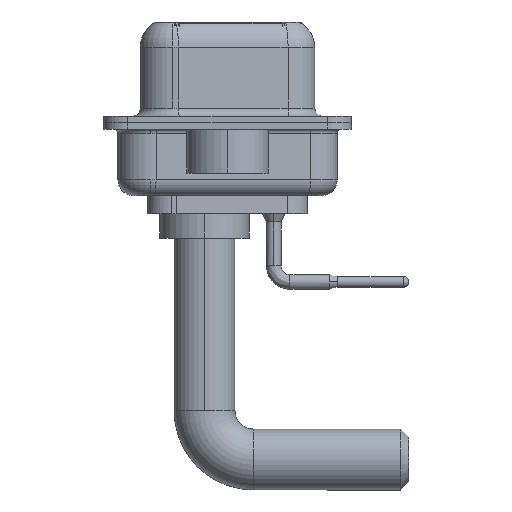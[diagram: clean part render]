
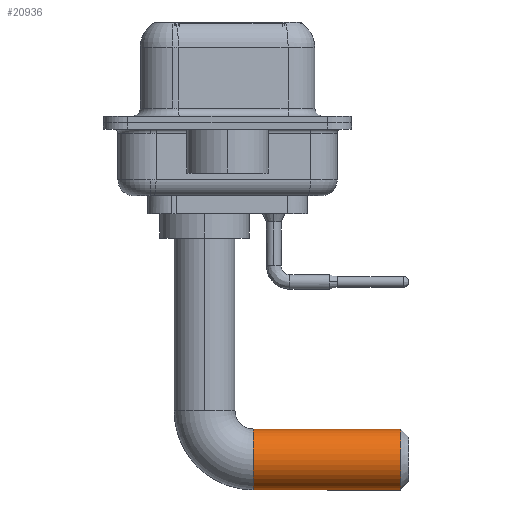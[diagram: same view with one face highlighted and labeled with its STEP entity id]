
A CAD part, left-side view. The second image highlights one B-rep face of the part: STEP entity #20936.
In plain terms, the highlighted cylindrical face has radius 1.875 mm (diameter 3.75 mm), a partial arc.
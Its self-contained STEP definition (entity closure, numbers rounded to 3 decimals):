
#50 = DIRECTION ( 'NONE',  ( -1., 0., 0. ) ) ;
#132 = EDGE_LOOP ( 'NONE', ( #13651, #15798, #13271, #6281 ) ) ;
#420 = CARTESIAN_POINT ( 'NONE',  ( 0., -3., -11.755 ) ) ;
#433 = LINE ( 'NONE', #12418, #16903 ) ;
#862 = AXIS2_PLACEMENT_3D ( 'NONE', #19703, #20893, #1698 ) ;
#1386 = CYLINDRICAL_SURFACE ( 'NONE', #862, 1.875 ) ;
#1459 = DIRECTION ( 'NONE',  ( 0., -1., 0. ) ) ;
#1698 = DIRECTION ( 'NONE',  ( 0., 0., -1. ) ) ;
#2107 = EDGE_CURVE ( 'NONE', #21097, #6196, #433, .T. ) ;
#2365 = EDGE_CURVE ( 'NONE', #9336, #9320, #11320, .T. ) ;
#3881 = CARTESIAN_POINT ( 'NONE',  ( 0., -12.07, -11.755 ) ) ;
#5141 = DIRECTION ( 'NONE',  ( 0., -1., 0. ) ) ;
#5563 = EDGE_CURVE ( 'NONE', #9320, #6196, #15329, .T. ) ;
#5795 = FACE_OUTER_BOUND ( 'NONE', #132, .T. ) ;
#6196 = VERTEX_POINT ( 'NONE', #3881 ) ;
#6281 = ORIENTED_EDGE ( 'NONE', *, *, #5563, .T. ) ;
#6403 = CIRCLE ( 'NONE', #9518, 1.875 ) ;
#9288 = CARTESIAN_POINT ( 'NONE',  ( 0., -3., -15.505 ) ) ;
#9320 = VERTEX_POINT ( 'NONE', #19049 ) ;
#9336 = VERTEX_POINT ( 'NONE', #9288 ) ;
#9518 = AXIS2_PLACEMENT_3D ( 'NONE', #14736, #9585, #50 ) ;
#9585 = DIRECTION ( 'NONE',  ( 0., -1., 0. ) ) ;
#10874 = AXIS2_PLACEMENT_3D ( 'NONE', #15949, #14142, #19469 ) ;
#11320 = LINE ( 'NONE', #16037, #14190 ) ;
#12178 = EDGE_CURVE ( 'NONE', #21097, #9336, #6403, .T. ) ;
#12418 = CARTESIAN_POINT ( 'NONE',  ( 0., -3., -11.755 ) ) ;
#13271 = ORIENTED_EDGE ( 'NONE', *, *, #2365, .T. ) ;
#13651 = ORIENTED_EDGE ( 'NONE', *, *, #2107, .F. ) ;
#14142 = DIRECTION ( 'NONE',  ( 0., 1., 0. ) ) ;
#14190 = VECTOR ( 'NONE', #1459, 1000. ) ;
#14736 = CARTESIAN_POINT ( 'NONE',  ( 0., -3., -13.63 ) ) ;
#15329 = CIRCLE ( 'NONE', #10874, 1.875 ) ;
#15798 = ORIENTED_EDGE ( 'NONE', *, *, #12178, .T. ) ;
#15949 = CARTESIAN_POINT ( 'NONE',  ( 0., -12.07, -13.63 ) ) ;
#16037 = CARTESIAN_POINT ( 'NONE',  ( 0., -3., -15.505 ) ) ;
#16903 = VECTOR ( 'NONE', #5141, 1000. ) ;
#19049 = CARTESIAN_POINT ( 'NONE',  ( 0., -12.07, -15.505 ) ) ;
#19469 = DIRECTION ( 'NONE',  ( 0., 0., -1. ) ) ;
#19703 = CARTESIAN_POINT ( 'NONE',  ( 0., -3., -13.63 ) ) ;
#20893 = DIRECTION ( 'NONE',  ( 0., -1., 0. ) ) ;
#20936 = ADVANCED_FACE ( 'NONE', ( #5795 ), #1386, .T. ) ;
#21097 = VERTEX_POINT ( 'NONE', #420 ) ;
